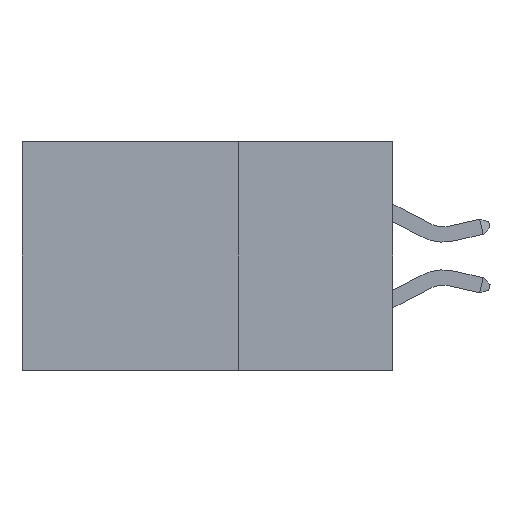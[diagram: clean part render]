
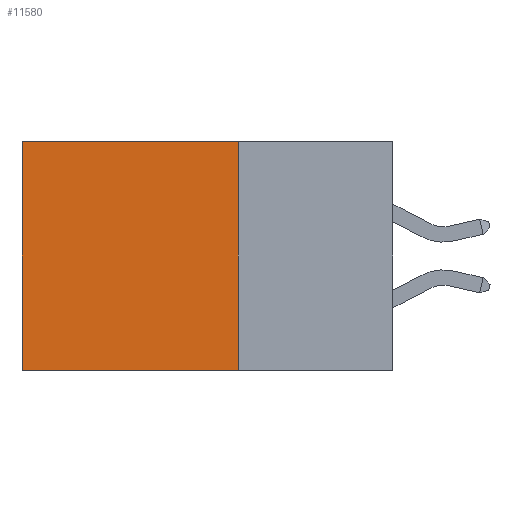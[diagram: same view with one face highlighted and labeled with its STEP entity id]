
A CAD part, left-side view. The second image highlights one B-rep face of the part: STEP entity #11580.
In plain terms, the highlighted planar face has unit normal (-1, 0, 0).
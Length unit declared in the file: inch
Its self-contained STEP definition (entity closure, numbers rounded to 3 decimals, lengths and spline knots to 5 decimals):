
#554 = VERTEX_POINT ( 'NONE', #6229 ) ;
#1258 = CARTESIAN_POINT ( 'NONE',  ( 0.2875, 0.25, 0. ) ) ;
#1529 = EDGE_CURVE ( 'NONE', #5060, #554, #8720, .T. ) ;
#1674 = DIRECTION ( 'NONE',  ( 0., 1., 0. ) ) ;
#1775 = FACE_OUTER_BOUND ( 'NONE', #6258, .T. ) ;
#2363 = VECTOR ( 'NONE', #1674, 39.37008 ) ;
#2641 = VECTOR ( 'NONE', #12198, 39.37008 ) ;
#2818 = CARTESIAN_POINT ( 'NONE',  ( 0.2875, 0.25, -0.37 ) ) ;
#4599 = DIRECTION ( 'NONE',  ( 0., 0., -1. ) ) ;
#4925 = ORIENTED_EDGE ( 'NONE', *, *, #12574, .T. ) ;
#5060 = VERTEX_POINT ( 'NONE', #12008 ) ;
#6229 = CARTESIAN_POINT ( 'NONE',  ( 0.2875, 0.6, 0. ) ) ;
#6258 = EDGE_LOOP ( 'NONE', ( #4925, #13050, #9377, #13245 ) ) ;
#6591 = PLANE ( 'NONE',  #13641 ) ;
#6688 = CARTESIAN_POINT ( 'NONE',  ( 0.2875, 0.25, 0. ) ) ;
#6974 = CARTESIAN_POINT ( 'NONE',  ( 0.2875, 0.6, 0. ) ) ;
#7442 = DIRECTION ( 'NONE',  ( 0., 0., -1. ) ) ;
#7908 = LINE ( 'NONE', #2818, #2641 ) ;
#8092 = LINE ( 'NONE', #6974, #13364 ) ;
#8720 = LINE ( 'NONE', #1258, #2363 ) ;
#9377 = ORIENTED_EDGE ( 'NONE', *, *, #11642, .F. ) ;
#9421 = VECTOR ( 'NONE', #7442, 39.37008 ) ;
#9649 = CARTESIAN_POINT ( 'NONE',  ( 0.2875, 0.6, -0.37 ) ) ;
#9736 = CARTESIAN_POINT ( 'NONE',  ( 0.2875, 0.25, -0.37 ) ) ;
#10080 = DIRECTION ( 'NONE',  ( 1., 0., 0. ) ) ;
#11000 = VERTEX_POINT ( 'NONE', #9736 ) ;
#11580 = ADVANCED_FACE ( 'NONE', ( #1775 ), #6591, .F. ) ;
#11642 = EDGE_CURVE ( 'NONE', #5060, #11000, #13383, .T. ) ;
#11972 = VERTEX_POINT ( 'NONE', #9649 ) ;
#12008 = CARTESIAN_POINT ( 'NONE',  ( 0.2875, 0.25, 0. ) ) ;
#12198 = DIRECTION ( 'NONE',  ( 0., 1., 0. ) ) ;
#12574 = EDGE_CURVE ( 'NONE', #554, #11972, #8092, .T. ) ;
#13050 = ORIENTED_EDGE ( 'NONE', *, *, #13481, .F. ) ;
#13245 = ORIENTED_EDGE ( 'NONE', *, *, #1529, .T. ) ;
#13364 = VECTOR ( 'NONE', #4599, 39.37008 ) ;
#13383 = LINE ( 'NONE', #13716, #9421 ) ;
#13481 = EDGE_CURVE ( 'NONE', #11000, #11972, #7908, .T. ) ;
#13641 = AXIS2_PLACEMENT_3D ( 'NONE', #6688, #10080, #14692 ) ;
#13716 = CARTESIAN_POINT ( 'NONE',  ( 0.2875, 0.25, 0. ) ) ;
#14692 = DIRECTION ( 'NONE',  ( 0., 0., -1. ) ) ;
